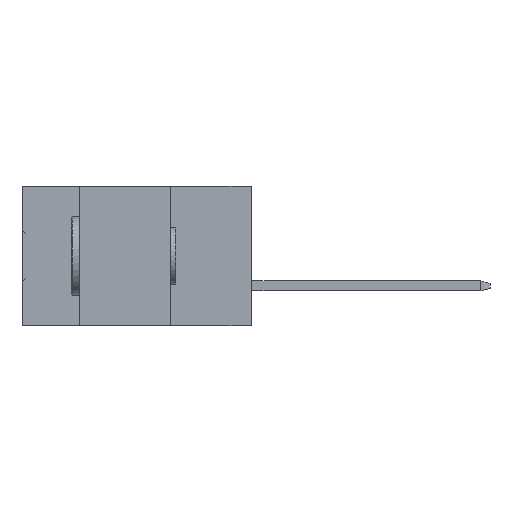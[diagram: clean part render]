
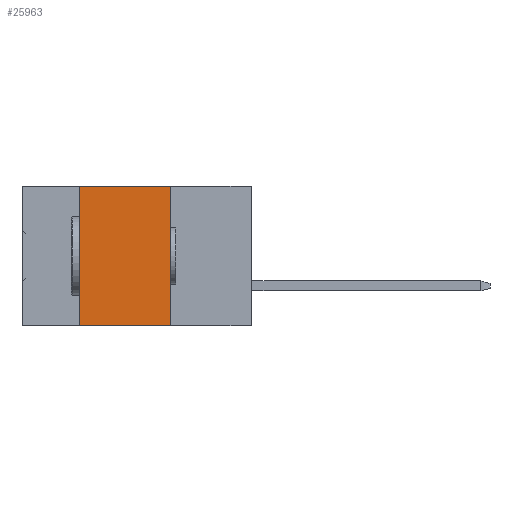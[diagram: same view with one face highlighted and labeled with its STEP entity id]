
A CAD part, left-side view. The second image highlights one B-rep face of the part: STEP entity #25963.
In plain terms, the highlighted planar face has unit normal (-1, 0, 0).
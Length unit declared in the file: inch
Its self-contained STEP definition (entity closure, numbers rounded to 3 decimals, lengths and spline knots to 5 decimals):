
#823 = CARTESIAN_POINT ( 'NONE',  ( 0., 0.254, -0.437 ) ) ;
#3604 = PLANE ( 'NONE',  #9540 ) ;
#5337 = DIRECTION ( 'NONE',  ( 0., -1., 0. ) ) ;
#6725 = EDGE_CURVE ( 'NONE', #27697, #19341, #26626, .T. ) ;
#8522 = DIRECTION ( 'NONE',  ( 0., 0., -1. ) ) ;
#8856 = ORIENTED_EDGE ( 'NONE', *, *, #9608, .F. ) ;
#9540 = AXIS2_PLACEMENT_3D ( 'NONE', #23036, #29855, #8522 ) ;
#9608 = EDGE_CURVE ( 'NONE', #27697, #23729, #19009, .T. ) ;
#9744 = CARTESIAN_POINT ( 'NONE',  ( 0., 0.254, 0. ) ) ;
#10295 = VECTOR ( 'NONE', #16693, 39.37008 ) ;
#11803 = CARTESIAN_POINT ( 'NONE',  ( 0., 0.54, -0.437 ) ) ;
#12608 = CARTESIAN_POINT ( 'NONE',  ( 0., 0.72, 0. ) ) ;
#12808 = EDGE_CURVE ( 'NONE', #18377, #19341, #24341, .T. ) ;
#14688 = CARTESIAN_POINT ( 'NONE',  ( 0., 0.54, 0. ) ) ;
#14929 = CARTESIAN_POINT ( 'NONE',  ( 0., 0.254, -0.437 ) ) ;
#15205 = DIRECTION ( 'NONE',  ( 0., -1., 0. ) ) ;
#15484 = VECTOR ( 'NONE', #5337, 39.37008 ) ;
#16237 = CARTESIAN_POINT ( 'NONE',  ( 0., 0.54, -0.437 ) ) ;
#16681 = ORIENTED_EDGE ( 'NONE', *, *, #12808, .F. ) ;
#16693 = DIRECTION ( 'NONE',  ( 0., 0., 1. ) ) ;
#18377 = VERTEX_POINT ( 'NONE', #9744 ) ;
#19009 = LINE ( 'NONE', #16237, #10295 ) ;
#19341 = VERTEX_POINT ( 'NONE', #823 ) ;
#20407 = FACE_OUTER_BOUND ( 'NONE', #24014, .T. ) ;
#21489 = VECTOR ( 'NONE', #24798, 39.37008 ) ;
#21620 = VECTOR ( 'NONE', #15205, 39.37008 ) ;
#23036 = CARTESIAN_POINT ( 'NONE',  ( 0., 0.72, 0. ) ) ;
#23729 = VERTEX_POINT ( 'NONE', #14688 ) ;
#24014 = EDGE_LOOP ( 'NONE', ( #16681, #30263, #8856, #26933 ) ) ;
#24167 = LINE ( 'NONE', #12608, #15484 ) ;
#24222 = EDGE_CURVE ( 'NONE', #23729, #18377, #24167, .T. ) ;
#24341 = LINE ( 'NONE', #14929, #21489 ) ;
#24798 = DIRECTION ( 'NONE',  ( 0., 0., -1. ) ) ;
#25963 = ADVANCED_FACE ( 'NONE', ( #20407 ), #3604, .F. ) ;
#26626 = LINE ( 'NONE', #26782, #21620 ) ;
#26782 = CARTESIAN_POINT ( 'NONE',  ( 0., 0.72, -0.437 ) ) ;
#26933 = ORIENTED_EDGE ( 'NONE', *, *, #6725, .T. ) ;
#27697 = VERTEX_POINT ( 'NONE', #11803 ) ;
#29855 = DIRECTION ( 'NONE',  ( 1., 0., 0. ) ) ;
#30263 = ORIENTED_EDGE ( 'NONE', *, *, #24222, .F. ) ;
